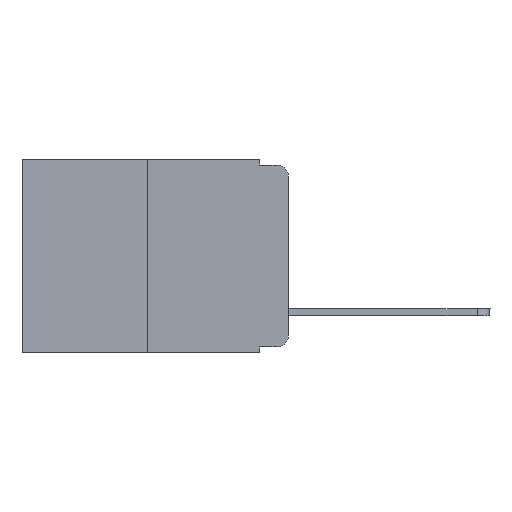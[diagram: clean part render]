
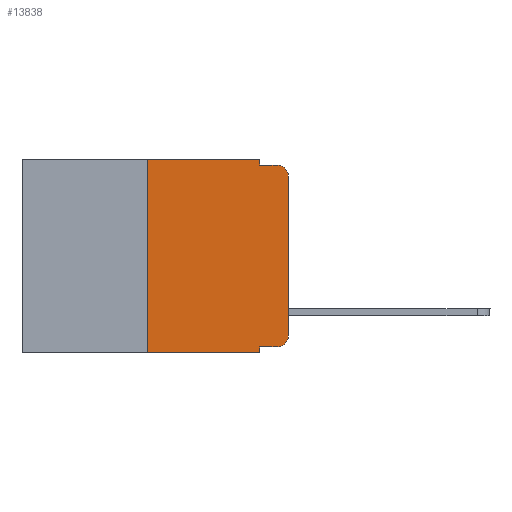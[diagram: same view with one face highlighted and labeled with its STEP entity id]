
A CAD part, left-side view. The second image highlights one B-rep face of the part: STEP entity #13838.
In plain terms, the highlighted planar face has unit normal (-1, 0, 0).
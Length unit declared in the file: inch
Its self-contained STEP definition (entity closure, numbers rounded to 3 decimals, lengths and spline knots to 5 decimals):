
#26 = DIRECTION ( 'NONE',  ( 0., 0., 1. ) ) ;
#72 = ORIENTED_EDGE ( 'NONE', *, *, #9726, .T. ) ;
#181 = AXIS2_PLACEMENT_3D ( 'NONE', #2264, #5714, #13877 ) ;
#194 = PLANE ( 'NONE',  #10550 ) ;
#617 = DIRECTION ( 'NONE',  ( 0., 0., -1. ) ) ;
#721 = LINE ( 'NONE', #14485, #3982 ) ;
#855 = ORIENTED_EDGE ( 'NONE', *, *, #9410, .T. ) ;
#994 = CARTESIAN_POINT ( 'NONE',  ( 0., 0.473, 0. ) ) ;
#1067 = FACE_OUTER_BOUND ( 'NONE', #1475, .T. ) ;
#1076 = CARTESIAN_POINT ( 'NONE',  ( 0., 0.051, -0.333 ) ) ;
#1240 = AXIS2_PLACEMENT_3D ( 'NONE', #3522, #6954, #1354 ) ;
#1334 = VECTOR ( 'NONE', #26, 39.37008 ) ;
#1354 = DIRECTION ( 'NONE',  ( 0., 0., -1. ) ) ;
#1475 = EDGE_LOOP ( 'NONE', ( #855, #3018, #2315, #4018, #8501, #7278, #72, #11983, #8161, #7723 ) ) ;
#1815 = EDGE_CURVE ( 'NONE', #6912, #2016, #10310, .T. ) ;
#2016 = VERTEX_POINT ( 'NONE', #13531 ) ;
#2264 = CARTESIAN_POINT ( 'NONE',  ( 0., 0.02, -0.313 ) ) ;
#2315 = ORIENTED_EDGE ( 'NONE', *, *, #12369, .F. ) ;
#2330 = EDGE_CURVE ( 'NONE', #9425, #13542, #721, .T. ) ;
#2374 = LINE ( 'NONE', #6940, #1334 ) ;
#2408 = CARTESIAN_POINT ( 'NONE',  ( 0., 0., 0. ) ) ;
#2481 = LINE ( 'NONE', #2408, #5391 ) ;
#2820 = CARTESIAN_POINT ( 'NONE',  ( 0., 0.02, -0.01 ) ) ;
#2899 = LINE ( 'NONE', #7455, #5800 ) ;
#3018 = ORIENTED_EDGE ( 'NONE', *, *, #11476, .T. ) ;
#3069 = LINE ( 'NONE', #11054, #10423 ) ;
#3125 = DIRECTION ( 'NONE',  ( 0., 0., -1. ) ) ;
#3522 = CARTESIAN_POINT ( 'NONE',  ( 0., 0.02, -0.03 ) ) ;
#3982 = VECTOR ( 'NONE', #13360, 39.37008 ) ;
#4018 = ORIENTED_EDGE ( 'NONE', *, *, #14198, .F. ) ;
#4196 = LINE ( 'NONE', #9867, #6983 ) ;
#4403 = CARTESIAN_POINT ( 'NONE',  ( 0., 0., -0.03 ) ) ;
#4561 = CARTESIAN_POINT ( 'NONE',  ( 0., 0.051, -0.333 ) ) ;
#5288 = CARTESIAN_POINT ( 'NONE',  ( 0., 0.25, -0.343 ) ) ;
#5391 = VECTOR ( 'NONE', #10485, 39.37008 ) ;
#5714 = DIRECTION ( 'NONE',  ( -1., 0., 0. ) ) ;
#5780 = CIRCLE ( 'NONE', #1240, 0.02 ) ;
#5800 = VECTOR ( 'NONE', #3125, 39.37008 ) ;
#5979 = VERTEX_POINT ( 'NONE', #2820 ) ;
#6053 = VERTEX_POINT ( 'NONE', #5288 ) ;
#6220 = VECTOR ( 'NONE', #9588, 39.37008 ) ;
#6274 = LINE ( 'NONE', #10610, #8944 ) ;
#6912 = VERTEX_POINT ( 'NONE', #1076 ) ;
#6940 = CARTESIAN_POINT ( 'NONE',  ( 0., 0.25, 0. ) ) ;
#6954 = DIRECTION ( 'NONE',  ( -1., 0., 0. ) ) ;
#6983 = VECTOR ( 'NONE', #14383, 39.37008 ) ;
#7278 = ORIENTED_EDGE ( 'NONE', *, *, #9047, .F. ) ;
#7455 = CARTESIAN_POINT ( 'NONE',  ( 0., 0.051, 0. ) ) ;
#7723 = ORIENTED_EDGE ( 'NONE', *, *, #9454, .T. ) ;
#7783 = DIRECTION ( 'NONE',  ( 0., 0., -1. ) ) ;
#8031 = CIRCLE ( 'NONE', #181, 0.02 ) ;
#8161 = ORIENTED_EDGE ( 'NONE', *, *, #1815, .T. ) ;
#8310 = EDGE_CURVE ( 'NONE', #6912, #10779, #6274, .T. ) ;
#8501 = ORIENTED_EDGE ( 'NONE', *, *, #2330, .F. ) ;
#8519 = VERTEX_POINT ( 'NONE', #11572 ) ;
#8941 = CARTESIAN_POINT ( 'NONE',  ( 0., 0.051, 0. ) ) ;
#8944 = VECTOR ( 'NONE', #617, 39.37008 ) ;
#8982 = DIRECTION ( 'NONE',  ( 1., 0., 0. ) ) ;
#9013 = VERTEX_POINT ( 'NONE', #4403 ) ;
#9047 = EDGE_CURVE ( 'NONE', #6053, #9425, #2374, .T. ) ;
#9410 = EDGE_CURVE ( 'NONE', #8519, #9013, #2481, .T. ) ;
#9425 = VERTEX_POINT ( 'NONE', #12481 ) ;
#9454 = EDGE_CURVE ( 'NONE', #2016, #8519, #8031, .T. ) ;
#9588 = DIRECTION ( 'NONE',  ( 0., -1., 0. ) ) ;
#9726 = EDGE_CURVE ( 'NONE', #6053, #10779, #3069, .T. ) ;
#9867 = CARTESIAN_POINT ( 'NONE',  ( 0., 0.051, -0.01 ) ) ;
#10310 = LINE ( 'NONE', #4561, #6220 ) ;
#10423 = VECTOR ( 'NONE', #14607, 39.37008 ) ;
#10485 = DIRECTION ( 'NONE',  ( 0., 0., 1. ) ) ;
#10550 = AXIS2_PLACEMENT_3D ( 'NONE', #994, #8982, #7783 ) ;
#10610 = CARTESIAN_POINT ( 'NONE',  ( 0., 0.051, 0. ) ) ;
#10779 = VERTEX_POINT ( 'NONE', #12172 ) ;
#11054 = CARTESIAN_POINT ( 'NONE',  ( 0., 0.473, -0.343 ) ) ;
#11476 = EDGE_CURVE ( 'NONE', #9013, #5979, #5780, .T. ) ;
#11572 = CARTESIAN_POINT ( 'NONE',  ( 0., 0., -0.313 ) ) ;
#11983 = ORIENTED_EDGE ( 'NONE', *, *, #8310, .F. ) ;
#12172 = CARTESIAN_POINT ( 'NONE',  ( 0., 0.051, -0.343 ) ) ;
#12369 = EDGE_CURVE ( 'NONE', #13836, #5979, #4196, .T. ) ;
#12460 = CARTESIAN_POINT ( 'NONE',  ( 0., 0.051, -0.01 ) ) ;
#12481 = CARTESIAN_POINT ( 'NONE',  ( 0., 0.25, 0. ) ) ;
#13360 = DIRECTION ( 'NONE',  ( 0., -1., 0. ) ) ;
#13531 = CARTESIAN_POINT ( 'NONE',  ( 0., 0.02, -0.333 ) ) ;
#13542 = VERTEX_POINT ( 'NONE', #8941 ) ;
#13836 = VERTEX_POINT ( 'NONE', #12460 ) ;
#13838 = ADVANCED_FACE ( 'NONE', ( #1067 ), #194, .F. ) ;
#13877 = DIRECTION ( 'NONE',  ( 0., 0., -1. ) ) ;
#14198 = EDGE_CURVE ( 'NONE', #13542, #13836, #2899, .T. ) ;
#14383 = DIRECTION ( 'NONE',  ( 0., -1., 0. ) ) ;
#14485 = CARTESIAN_POINT ( 'NONE',  ( 0., 0.473, 0. ) ) ;
#14607 = DIRECTION ( 'NONE',  ( 0., -1., 0. ) ) ;
